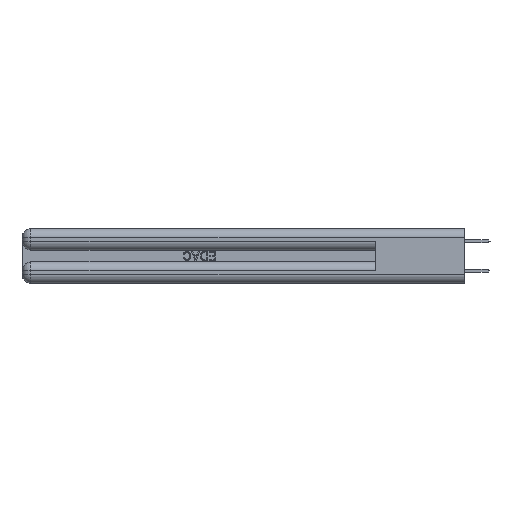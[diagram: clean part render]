
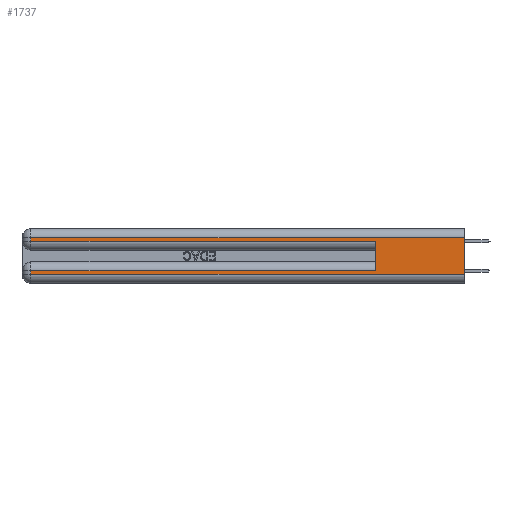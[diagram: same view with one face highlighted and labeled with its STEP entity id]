
A CAD part, left-side view. The second image highlights one B-rep face of the part: STEP entity #1737.
In plain terms, the highlighted planar face has unit normal (-1, 0, 0).
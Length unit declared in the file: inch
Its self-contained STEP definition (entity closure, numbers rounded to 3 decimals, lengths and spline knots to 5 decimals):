
#196 = ORIENTED_EDGE ( 'NONE', *, *, #2435, .T. ) ;
#1737 = ADVANCED_FACE ( 'NONE', ( #24246 ), #20179, .F. ) ;
#2435 = EDGE_CURVE ( 'NONE', #25187, #40453, #41790, .T. ) ;
#3913 = VECTOR ( 'NONE', #6162, 39.37008 ) ;
#4599 = CARTESIAN_POINT ( 'NONE',  ( 0., 0.6, 0.085 ) ) ;
#4705 = CARTESIAN_POINT ( 'NONE',  ( 0., 0., 0.285 ) ) ;
#5325 = VERTEX_POINT ( 'NONE', #11257 ) ;
#5625 = VERTEX_POINT ( 'NONE', #34372 ) ;
#5770 = AXIS2_PLACEMENT_3D ( 'NONE', #14045, #13919, #30120 ) ;
#6024 = VECTOR ( 'NONE', #41107, 39.37008 ) ;
#6162 = DIRECTION ( 'NONE',  ( 0., 0., 1. ) ) ;
#8072 = CARTESIAN_POINT ( 'NONE',  ( 0., 0., 0.31 ) ) ;
#8437 = EDGE_CURVE ( 'NONE', #14280, #5325, #35845, .T. ) ;
#8632 = DIRECTION ( 'NONE',  ( 0., 0., -1. ) ) ;
#11127 = DIRECTION ( 'NONE',  ( 0., -1., 0. ) ) ;
#11257 = CARTESIAN_POINT ( 'NONE',  ( 0., 2.94, 0.085 ) ) ;
#11703 = LINE ( 'NONE', #12729, #23113 ) ;
#11742 = VERTEX_POINT ( 'NONE', #16798 ) ;
#12477 = LINE ( 'NONE', #41423, #19742 ) ;
#12594 = CARTESIAN_POINT ( 'NONE',  ( 0., 2.94, 0.37 ) ) ;
#12729 = CARTESIAN_POINT ( 'NONE',  ( 0., 0., 0.31 ) ) ;
#13088 = CARTESIAN_POINT ( 'NONE',  ( 0., 0.6, 0.145 ) ) ;
#13919 = DIRECTION ( 'NONE',  ( 1., 0., 0. ) ) ;
#14045 = CARTESIAN_POINT ( 'NONE',  ( 0., 0., 0.37 ) ) ;
#14280 = VERTEX_POINT ( 'NONE', #4599 ) ;
#14964 = EDGE_CURVE ( 'NONE', #14280, #15292, #22059, .T. ) ;
#15016 = EDGE_CURVE ( 'NONE', #18221, #25187, #11703, .T. ) ;
#15292 = VERTEX_POINT ( 'NONE', #18625 ) ;
#16798 = CARTESIAN_POINT ( 'NONE',  ( 0., 2.94, 0.06 ) ) ;
#17418 = ORIENTED_EDGE ( 'NONE', *, *, #33648, .T. ) ;
#18221 = VERTEX_POINT ( 'NONE', #8072 ) ;
#18625 = CARTESIAN_POINT ( 'NONE',  ( 0., 0.6, 0.285 ) ) ;
#18641 = ORIENTED_EDGE ( 'NONE', *, *, #15016, .T. ) ;
#19742 = VECTOR ( 'NONE', #8632, 39.37008 ) ;
#19846 = VECTOR ( 'NONE', #31202, 39.37008 ) ;
#20179 = PLANE ( 'NONE',  #5770 ) ;
#22059 = LINE ( 'NONE', #13088, #3913 ) ;
#22262 = DIRECTION ( 'NONE',  ( 0., 1., 0. ) ) ;
#23113 = VECTOR ( 'NONE', #22262, 39.37008 ) ;
#23137 = LINE ( 'NONE', #4705, #6024 ) ;
#24246 = FACE_OUTER_BOUND ( 'NONE', #26773, .T. ) ;
#24263 = VECTOR ( 'NONE', #41176, 39.37008 ) ;
#24429 = CARTESIAN_POINT ( 'NONE',  ( 0., 0., 0.06 ) ) ;
#24637 = ORIENTED_EDGE ( 'NONE', *, *, #8437, .T. ) ;
#24669 = VECTOR ( 'NONE', #11127, 39.37008 ) ;
#25187 = VERTEX_POINT ( 'NONE', #25937 ) ;
#25937 = CARTESIAN_POINT ( 'NONE',  ( 0., 2.94, 0.31 ) ) ;
#26101 = EDGE_CURVE ( 'NONE', #40453, #15292, #23137, .T. ) ;
#26487 = DIRECTION ( 'NONE',  ( 0., 0., -1. ) ) ;
#26773 = EDGE_LOOP ( 'NONE', ( #35116, #18641, #196, #41334, #34915, #24637, #17418, #42128 ) ) ;
#28583 = CARTESIAN_POINT ( 'NONE',  ( 0., 2.94, 0.285 ) ) ;
#30120 = DIRECTION ( 'NONE',  ( 0., 0., -1. ) ) ;
#31202 = DIRECTION ( 'NONE',  ( 0., 1., 0. ) ) ;
#32994 = LINE ( 'NONE', #24429, #24669 ) ;
#33648 = EDGE_CURVE ( 'NONE', #5325, #11742, #34093, .T. ) ;
#34026 = VECTOR ( 'NONE', #26487, 39.37008 ) ;
#34093 = LINE ( 'NONE', #37561, #24263 ) ;
#34211 = CARTESIAN_POINT ( 'NONE',  ( 0., 0., 0.085 ) ) ;
#34372 = CARTESIAN_POINT ( 'NONE',  ( 0., 0., 0.06 ) ) ;
#34915 = ORIENTED_EDGE ( 'NONE', *, *, #14964, .F. ) ;
#35116 = ORIENTED_EDGE ( 'NONE', *, *, #36488, .F. ) ;
#35845 = LINE ( 'NONE', #34211, #19846 ) ;
#36488 = EDGE_CURVE ( 'NONE', #18221, #5625, #12477, .T. ) ;
#37561 = CARTESIAN_POINT ( 'NONE',  ( 0., 2.94, 0.37 ) ) ;
#38847 = EDGE_CURVE ( 'NONE', #11742, #5625, #32994, .T. ) ;
#40453 = VERTEX_POINT ( 'NONE', #28583 ) ;
#41107 = DIRECTION ( 'NONE',  ( 0., -1., 0. ) ) ;
#41176 = DIRECTION ( 'NONE',  ( 0., 0., -1. ) ) ;
#41334 = ORIENTED_EDGE ( 'NONE', *, *, #26101, .T. ) ;
#41423 = CARTESIAN_POINT ( 'NONE',  ( 0., 0., 0.37 ) ) ;
#41790 = LINE ( 'NONE', #12594, #34026 ) ;
#42128 = ORIENTED_EDGE ( 'NONE', *, *, #38847, .T. ) ;
